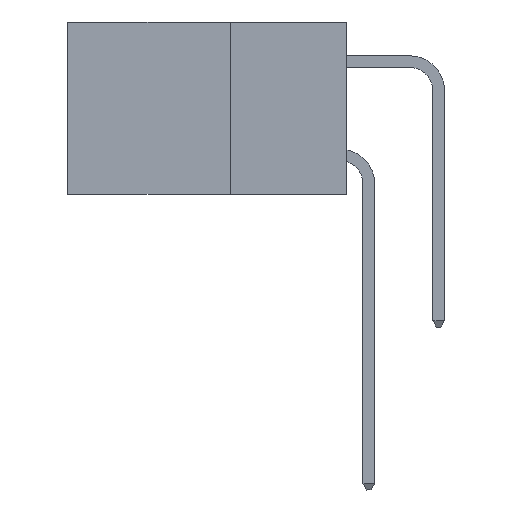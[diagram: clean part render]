
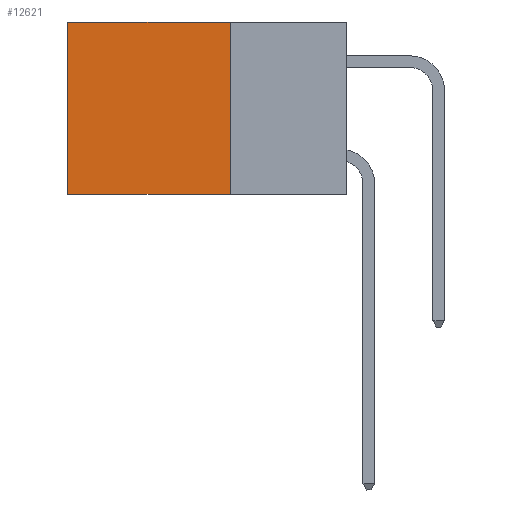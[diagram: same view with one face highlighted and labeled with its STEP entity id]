
A CAD part, left-side view. The second image highlights one B-rep face of the part: STEP entity #12621.
In plain terms, the highlighted planar face has unit normal (-1, 0, 0).
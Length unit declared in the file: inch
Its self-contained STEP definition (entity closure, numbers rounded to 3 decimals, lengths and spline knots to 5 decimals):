
#42 = EDGE_CURVE ( 'NONE', #8906, #12633, #10589, .T. ) ;
#169 = CARTESIAN_POINT ( 'NONE',  ( 0.2875, 0.6, 0. ) ) ;
#308 = DIRECTION ( 'NONE',  ( 0., 1., 0. ) ) ;
#669 = ORIENTED_EDGE ( 'NONE', *, *, #42, .F. ) ;
#1264 = CARTESIAN_POINT ( 'NONE',  ( 0.2875, 0.25, 0. ) ) ;
#1447 = CARTESIAN_POINT ( 'NONE',  ( 0.2875, 0.25, 0. ) ) ;
#2009 = CARTESIAN_POINT ( 'NONE',  ( 0.2875, 0.25, 0. ) ) ;
#2485 = PLANE ( 'NONE',  #11832 ) ;
#2926 = VERTEX_POINT ( 'NONE', #2009 ) ;
#3099 = EDGE_CURVE ( 'NONE', #2926, #4122, #12457, .T. ) ;
#3452 = DIRECTION ( 'NONE',  ( 0., 0., -1. ) ) ;
#4122 = VERTEX_POINT ( 'NONE', #9038 ) ;
#4247 = FACE_OUTER_BOUND ( 'NONE', #10510, .T. ) ;
#4530 = ORIENTED_EDGE ( 'NONE', *, *, #5759, .T. ) ;
#4564 = DIRECTION ( 'NONE',  ( 0., 1., 0. ) ) ;
#4910 = CARTESIAN_POINT ( 'NONE',  ( 0.2875, 0.25, -0.37 ) ) ;
#5306 = VECTOR ( 'NONE', #7445, 39.37008 ) ;
#5584 = ORIENTED_EDGE ( 'NONE', *, *, #3099, .T. ) ;
#5759 = EDGE_CURVE ( 'NONE', #4122, #12633, #12985, .T. ) ;
#7030 = VECTOR ( 'NONE', #308, 39.37008 ) ;
#7445 = DIRECTION ( 'NONE',  ( 0., 0., -1. ) ) ;
#7497 = CARTESIAN_POINT ( 'NONE',  ( 0.2875, 0.25, 0. ) ) ;
#7876 = VECTOR ( 'NONE', #4564, 39.37008 ) ;
#8906 = VERTEX_POINT ( 'NONE', #4910 ) ;
#9038 = CARTESIAN_POINT ( 'NONE',  ( 0.2875, 0.6, 0. ) ) ;
#9171 = EDGE_CURVE ( 'NONE', #2926, #8906, #10353, .T. ) ;
#9562 = DIRECTION ( 'NONE',  ( 1., 0., 0. ) ) ;
#10298 = VECTOR ( 'NONE', #12308, 39.37008 ) ;
#10353 = LINE ( 'NONE', #1447, #5306 ) ;
#10389 = CARTESIAN_POINT ( 'NONE',  ( 0.2875, 0.25, -0.37 ) ) ;
#10510 = EDGE_LOOP ( 'NONE', ( #4530, #669, #10620, #5584 ) ) ;
#10589 = LINE ( 'NONE', #10389, #7876 ) ;
#10620 = ORIENTED_EDGE ( 'NONE', *, *, #9171, .F. ) ;
#11832 = AXIS2_PLACEMENT_3D ( 'NONE', #7497, #9562, #3452 ) ;
#12308 = DIRECTION ( 'NONE',  ( 0., 0., -1. ) ) ;
#12457 = LINE ( 'NONE', #1264, #7030 ) ;
#12586 = CARTESIAN_POINT ( 'NONE',  ( 0.2875, 0.6, -0.37 ) ) ;
#12621 = ADVANCED_FACE ( 'NONE', ( #4247 ), #2485, .F. ) ;
#12633 = VERTEX_POINT ( 'NONE', #12586 ) ;
#12985 = LINE ( 'NONE', #169, #10298 ) ;
